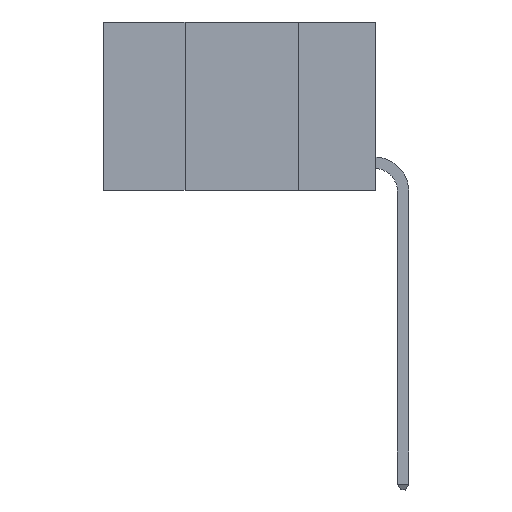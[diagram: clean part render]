
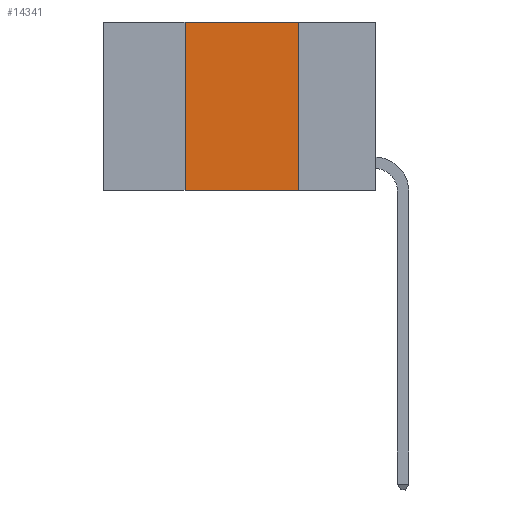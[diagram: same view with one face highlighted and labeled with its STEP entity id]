
A CAD part, left-side view. The second image highlights one B-rep face of the part: STEP entity #14341.
In plain terms, the highlighted planar face has unit normal (-1, 0, 0).
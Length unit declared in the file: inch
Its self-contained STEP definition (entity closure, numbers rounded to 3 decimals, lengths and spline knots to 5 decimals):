
#658 = CARTESIAN_POINT ( 'NONE',  ( 0., 0.6, 0. ) ) ;
#1039 = CARTESIAN_POINT ( 'NONE',  ( 0., 0.42, 0. ) ) ;
#1066 = CARTESIAN_POINT ( 'NONE',  ( 0., 0.42, -0.37 ) ) ;
#1110 = DIRECTION ( 'NONE',  ( 0., -1., 0. ) ) ;
#1218 = ORIENTED_EDGE ( 'NONE', *, *, #8044, .T. ) ;
#1723 = LINE ( 'NONE', #1039, #9014 ) ;
#2024 = LINE ( 'NONE', #15345, #9322 ) ;
#2035 = VERTEX_POINT ( 'NONE', #9169 ) ;
#2113 = VECTOR ( 'NONE', #16632, 39.37008 ) ;
#2776 = LINE ( 'NONE', #17536, #5564 ) ;
#3396 = VERTEX_POINT ( 'NONE', #6747 ) ;
#3432 = DIRECTION ( 'NONE',  ( 0., 0., -1. ) ) ;
#4670 = FACE_OUTER_BOUND ( 'NONE', #5321, .T. ) ;
#4924 = LINE ( 'NONE', #7053, #2113 ) ;
#5130 = DIRECTION ( 'NONE',  ( 0., 0., 1. ) ) ;
#5234 = EDGE_CURVE ( 'NONE', #3396, #2035, #2776, .T. ) ;
#5321 = EDGE_LOOP ( 'NONE', ( #10295, #10980, #12544, #1218 ) ) ;
#5564 = VECTOR ( 'NONE', #1110, 39.37008 ) ;
#6747 = CARTESIAN_POINT ( 'NONE',  ( 0., 0.42, 0. ) ) ;
#7053 = CARTESIAN_POINT ( 'NONE',  ( 0., 0.17, 0. ) ) ;
#7156 = DIRECTION ( 'NONE',  ( 0., -1., 0. ) ) ;
#8044 = EDGE_CURVE ( 'NONE', #12717, #8298, #2024, .T. ) ;
#8298 = VERTEX_POINT ( 'NONE', #9018 ) ;
#9014 = VECTOR ( 'NONE', #5130, 39.37008 ) ;
#9018 = CARTESIAN_POINT ( 'NONE',  ( 0., 0.17, -0.37 ) ) ;
#9169 = CARTESIAN_POINT ( 'NONE',  ( 0., 0.17, 0. ) ) ;
#9322 = VECTOR ( 'NONE', #7156, 39.37008 ) ;
#10255 = PLANE ( 'NONE',  #11010 ) ;
#10295 = ORIENTED_EDGE ( 'NONE', *, *, #16413, .F. ) ;
#10980 = ORIENTED_EDGE ( 'NONE', *, *, #5234, .F. ) ;
#11010 = AXIS2_PLACEMENT_3D ( 'NONE', #658, #11615, #3432 ) ;
#11615 = DIRECTION ( 'NONE',  ( 1., 0., 0. ) ) ;
#12544 = ORIENTED_EDGE ( 'NONE', *, *, #15477, .F. ) ;
#12717 = VERTEX_POINT ( 'NONE', #1066 ) ;
#14341 = ADVANCED_FACE ( 'NONE', ( #4670 ), #10255, .F. ) ;
#15345 = CARTESIAN_POINT ( 'NONE',  ( 0., 0.6, -0.37 ) ) ;
#15477 = EDGE_CURVE ( 'NONE', #12717, #3396, #1723, .T. ) ;
#16413 = EDGE_CURVE ( 'NONE', #2035, #8298, #4924, .T. ) ;
#16632 = DIRECTION ( 'NONE',  ( 0., 0., -1. ) ) ;
#17536 = CARTESIAN_POINT ( 'NONE',  ( 0., 0.6, 0. ) ) ;
